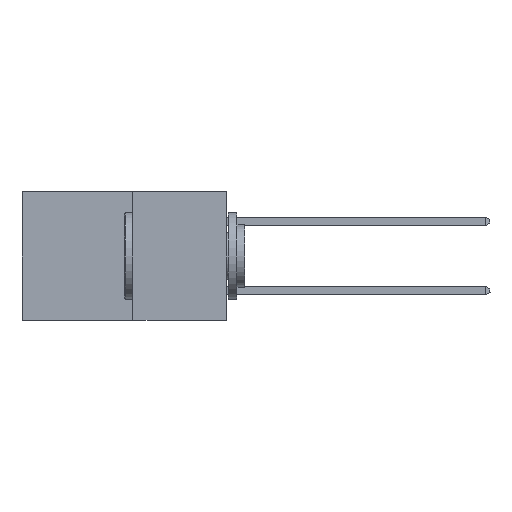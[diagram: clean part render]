
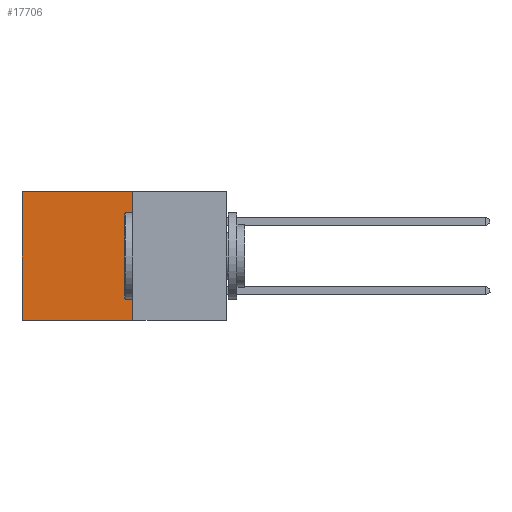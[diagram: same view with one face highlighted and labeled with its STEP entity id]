
A CAD part, left-side view. The second image highlights one B-rep face of the part: STEP entity #17706.
In plain terms, the highlighted planar face has unit normal (-1, 0, 0).
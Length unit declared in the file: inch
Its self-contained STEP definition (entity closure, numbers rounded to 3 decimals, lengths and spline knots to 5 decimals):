
#611 = DIRECTION ( 'NONE',  ( 0., 0., -1. ) ) ;
#2045 = CARTESIAN_POINT ( 'NONE',  ( 0.277, 0.27, -0.37 ) ) ;
#2445 = CARTESIAN_POINT ( 'NONE',  ( 0.277, 0.27, -0.37 ) ) ;
#2753 = EDGE_CURVE ( 'NONE', #13374, #9419, #23183, .T. ) ;
#3045 = CARTESIAN_POINT ( 'NONE',  ( 0.277, 0.27, -0.37 ) ) ;
#3871 = PLANE ( 'NONE',  #17143 ) ;
#3914 = ORIENTED_EDGE ( 'NONE', *, *, #2753, .T. ) ;
#4948 = CARTESIAN_POINT ( 'NONE',  ( 0.277, 0.59, -0.37 ) ) ;
#5955 = VERTEX_POINT ( 'NONE', #8190 ) ;
#5962 = EDGE_CURVE ( 'NONE', #5955, #13374, #22362, .T. ) ;
#7446 = EDGE_CURVE ( 'NONE', #13071, #9419, #10693, .T. ) ;
#8190 = CARTESIAN_POINT ( 'NONE',  ( 0.277, 0.27, 0. ) ) ;
#8601 = ORIENTED_EDGE ( 'NONE', *, *, #23794, .F. ) ;
#9419 = VERTEX_POINT ( 'NONE', #4948 ) ;
#9593 = VECTOR ( 'NONE', #16096, 39.37008 ) ;
#10535 = EDGE_LOOP ( 'NONE', ( #3914, #16101, #8601, #19900 ) ) ;
#10693 = LINE ( 'NONE', #3045, #19958 ) ;
#11929 = CARTESIAN_POINT ( 'NONE',  ( 0.277, 0.27, 0. ) ) ;
#12075 = FACE_OUTER_BOUND ( 'NONE', #10535, .T. ) ;
#13071 = VERTEX_POINT ( 'NONE', #2445 ) ;
#13374 = VERTEX_POINT ( 'NONE', #21726 ) ;
#15569 = DIRECTION ( 'NONE',  ( 0., 1., 0. ) ) ;
#15964 = DIRECTION ( 'NONE',  ( 0., 1., 0. ) ) ;
#16096 = DIRECTION ( 'NONE',  ( 0., 0., -1. ) ) ;
#16101 = ORIENTED_EDGE ( 'NONE', *, *, #7446, .F. ) ;
#16793 = DIRECTION ( 'NONE',  ( 0., 0., -1. ) ) ;
#17143 = AXIS2_PLACEMENT_3D ( 'NONE', #2045, #22317, #16793 ) ;
#17175 = CARTESIAN_POINT ( 'NONE',  ( 0.277, 0.27, -0.37 ) ) ;
#17431 = VECTOR ( 'NONE', #15569, 39.37008 ) ;
#17706 = ADVANCED_FACE ( 'NONE', ( #12075 ), #3871, .F. ) ;
#19900 = ORIENTED_EDGE ( 'NONE', *, *, #5962, .T. ) ;
#19923 = VECTOR ( 'NONE', #611, 39.37008 ) ;
#19958 = VECTOR ( 'NONE', #15964, 39.37008 ) ;
#20187 = CARTESIAN_POINT ( 'NONE',  ( 0.277, 0.59, -0.37 ) ) ;
#20508 = LINE ( 'NONE', #17175, #19923 ) ;
#21726 = CARTESIAN_POINT ( 'NONE',  ( 0.277, 0.59, 0. ) ) ;
#22317 = DIRECTION ( 'NONE',  ( 1., 0., 0. ) ) ;
#22362 = LINE ( 'NONE', #11929, #17431 ) ;
#23183 = LINE ( 'NONE', #20187, #9593 ) ;
#23794 = EDGE_CURVE ( 'NONE', #5955, #13071, #20508, .T. ) ;
